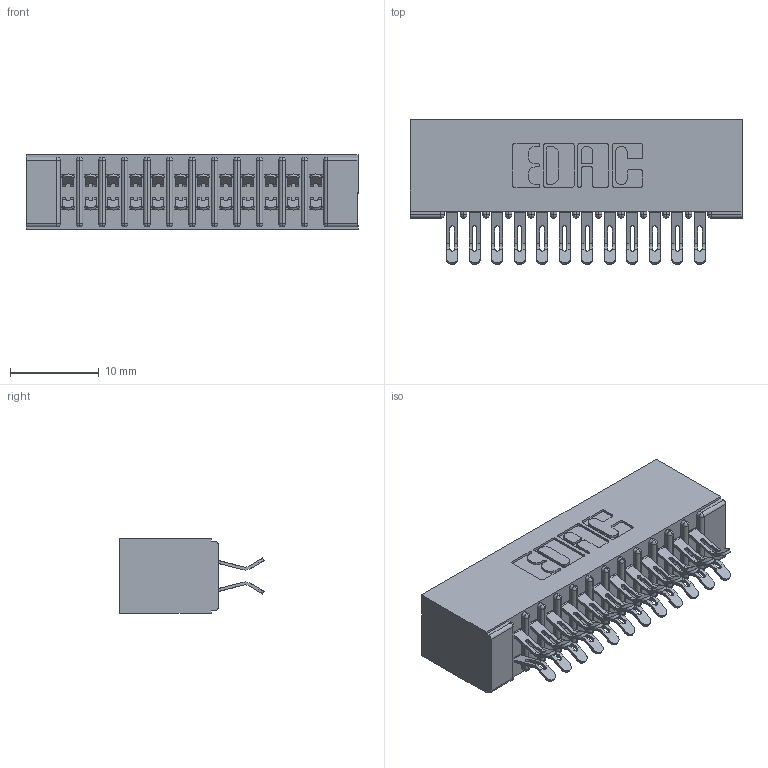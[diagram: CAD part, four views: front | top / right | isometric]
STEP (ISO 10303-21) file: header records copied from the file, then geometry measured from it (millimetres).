
FILE_DESCRIPTION (( 'STEP AP203' ), '1' );
FILE_NAME ('341-024-555-201.STEP', '2018-08-06T18:09:41', ( '' ), ( '' ), 'SwSTEP 2.0', 'SolidWorks 2016', '' );
FILE_SCHEMA (( 'CONFIG_CONTROL_DESIGN' ));
Length unit declared in the file: inch
Products named in the file (3): 341-292-001_341-292-155; 341-024-555-201; 341 Part_No Mounting Lugs
Assembly tree (25 placements, depth 2):
  341-024-555-201
    341 Part_No Mounting Lugs
    341-292-001_341-292-155  x24
Bounding box: 37.47 x 16.31 x 8.38 mm (x, y, z)
Volume: 2319.5 mm3; surface area: 5078 mm2
Topology: 25 solids, 25 shells, 1980 faces, 5896 edges, 3838 vertices
Faces by surface type: plane 1072, cylinder 860, sphere 26, torus 22
Entity records: 18711 total; most frequent: CARTESIAN_POINT 3126, ORIENTED_EDGE 3092, DIRECTION 3044, EDGE_CURVE 1546, VECTOR 1204, LINE 1204, VERTEX_POINT 986, AXIS2_PLACEMENT_3D 920
